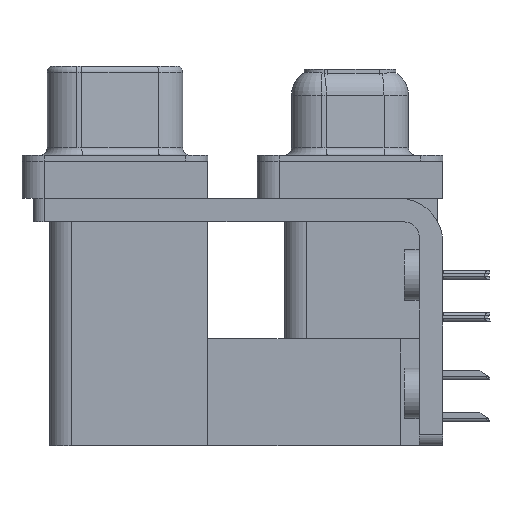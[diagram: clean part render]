
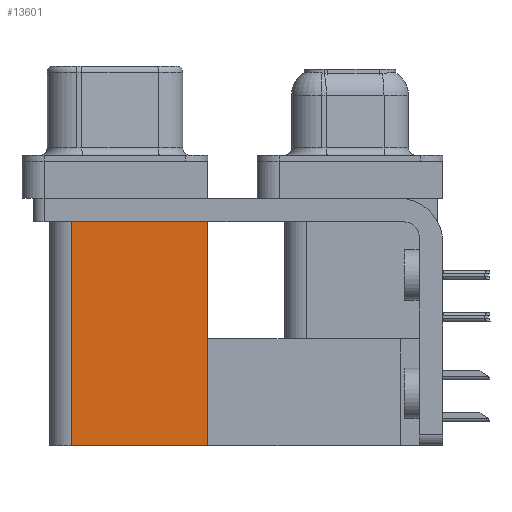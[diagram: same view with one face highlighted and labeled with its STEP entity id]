
A CAD part, left-side view. The second image highlights one B-rep face of the part: STEP entity #13601.
In plain terms, the highlighted planar face has unit normal (-1, 0, 0).
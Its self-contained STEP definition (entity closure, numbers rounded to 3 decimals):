
#433 = ORIENTED_EDGE ( 'NONE', *, *, #13713, .F. ) ;
#1292 = CARTESIAN_POINT ( 'NONE',  ( 3.765, 18.8, -19.2 ) ) ;
#1794 = VERTEX_POINT ( 'NONE', #1292 ) ;
#2741 = VECTOR ( 'NONE', #43710, 1000. ) ;
#5708 = VECTOR ( 'NONE', #45516, 1000. ) ;
#6159 = LINE ( 'NONE', #34878, #20512 ) ;
#7129 = ORIENTED_EDGE ( 'NONE', *, *, #18740, .T. ) ;
#7310 = VERTEX_POINT ( 'NONE', #42399 ) ;
#7912 = EDGE_CURVE ( 'NONE', #7310, #26914, #9304, .T. ) ;
#9304 = LINE ( 'NONE', #24371, #5708 ) ;
#11025 = VECTOR ( 'NONE', #29029, 1000. ) ;
#13511 = EDGE_LOOP ( 'NONE', ( #32041, #22144, #433, #7129 ) ) ;
#13601 = ADVANCED_FACE ( 'NONE', ( #38634 ), #23837, .F. ) ;
#13697 = DIRECTION ( 'NONE',  ( 1., 0., 0. ) ) ;
#13713 = EDGE_CURVE ( 'NONE', #30481, #1794, #6159, .T. ) ;
#14496 = CARTESIAN_POINT ( 'NONE',  ( 3.765, 18.8, -2.5 ) ) ;
#15958 = AXIS2_PLACEMENT_3D ( 'NONE', #38160, #13697, #35108 ) ;
#18740 = EDGE_CURVE ( 'NONE', #30481, #7310, #29479, .T. ) ;
#20512 = VECTOR ( 'NONE', #35337, 1000. ) ;
#22144 = ORIENTED_EDGE ( 'NONE', *, *, #41754, .F. ) ;
#23786 = CARTESIAN_POINT ( 'NONE',  ( 3.765, 9.6, -19.2 ) ) ;
#23837 = PLANE ( 'NONE',  #15958 ) ;
#24371 = CARTESIAN_POINT ( 'NONE',  ( 3.765, 9.6, -2.5 ) ) ;
#26914 = VERTEX_POINT ( 'NONE', #14496 ) ;
#29029 = DIRECTION ( 'NONE',  ( 0., 0., 1. ) ) ;
#29259 = CARTESIAN_POINT ( 'NONE',  ( 3.765, 9.6, -19.2 ) ) ;
#29479 = LINE ( 'NONE', #29259, #11025 ) ;
#30481 = VERTEX_POINT ( 'NONE', #23786 ) ;
#32041 = ORIENTED_EDGE ( 'NONE', *, *, #7912, .T. ) ;
#33589 = LINE ( 'NONE', #43940, #2741 ) ;
#34878 = CARTESIAN_POINT ( 'NONE',  ( 3.765, 9.6, -19.2 ) ) ;
#35108 = DIRECTION ( 'NONE',  ( 0., 0., -1. ) ) ;
#35337 = DIRECTION ( 'NONE',  ( 0., 1., 0. ) ) ;
#38160 = CARTESIAN_POINT ( 'NONE',  ( 3.765, 9.6, -19.2 ) ) ;
#38634 = FACE_OUTER_BOUND ( 'NONE', #13511, .T. ) ;
#41754 = EDGE_CURVE ( 'NONE', #1794, #26914, #33589, .T. ) ;
#42399 = CARTESIAN_POINT ( 'NONE',  ( 3.765, 9.6, -2.5 ) ) ;
#43710 = DIRECTION ( 'NONE',  ( 0., 0., 1. ) ) ;
#43940 = CARTESIAN_POINT ( 'NONE',  ( 3.765, 18.8, -19.2 ) ) ;
#45516 = DIRECTION ( 'NONE',  ( 0., 1., 0. ) ) ;
